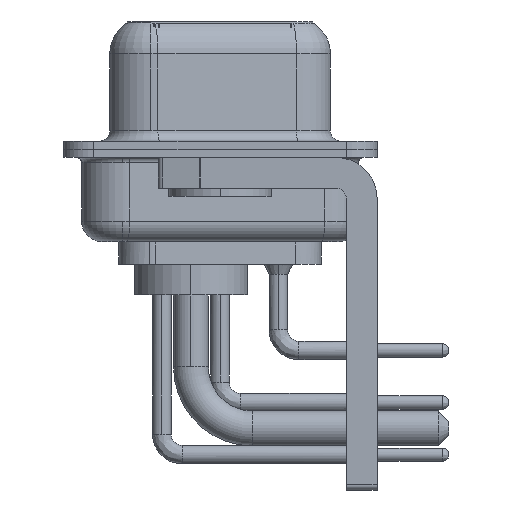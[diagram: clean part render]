
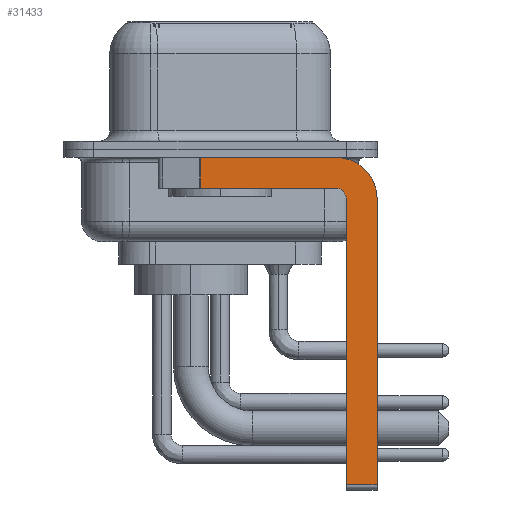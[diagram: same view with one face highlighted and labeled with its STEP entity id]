
A CAD part, left-side view. The second image highlights one B-rep face of the part: STEP entity #31433.
In plain terms, the highlighted planar face has unit normal (-1, 0, 0).
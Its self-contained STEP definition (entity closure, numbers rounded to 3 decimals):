
#426 = ORIENTED_EDGE ( 'NONE', *, *, #25855, .F. ) ;
#1283 = DIRECTION ( 'NONE',  ( 1., 0., 0. ) ) ;
#1413 = CARTESIAN_POINT ( 'NONE',  ( -2.9, 0.978, -1.9 ) ) ;
#2458 = LINE ( 'NONE', #3112, #21008 ) ;
#2875 = CIRCLE ( 'NONE', #27595, 0.5 ) ;
#3047 = CARTESIAN_POINT ( 'NONE',  ( -2.9, -5.65, -0.4 ) ) ;
#3112 = CARTESIAN_POINT ( 'NONE',  ( -2.9, -5.65, -1.9 ) ) ;
#3438 = DIRECTION ( 'NONE',  ( 1., 0., 0. ) ) ;
#4174 = LINE ( 'NONE', #7235, #6791 ) ;
#4279 = VERTEX_POINT ( 'NONE', #17895 ) ;
#5660 = CARTESIAN_POINT ( 'NONE',  ( -2.9, 0.978, -1.9 ) ) ;
#6791 = VECTOR ( 'NONE', #12461, 1000. ) ;
#7014 = ORIENTED_EDGE ( 'NONE', *, *, #28611, .F. ) ;
#7235 = CARTESIAN_POINT ( 'NONE',  ( -2.9, 3., -0.4 ) ) ;
#7258 = ORIENTED_EDGE ( 'NONE', *, *, #32996, .F. ) ;
#8480 = ORIENTED_EDGE ( 'NONE', *, *, #21871, .F. ) ;
#8624 = VERTEX_POINT ( 'NONE', #5660 ) ;
#8883 = EDGE_CURVE ( 'NONE', #15391, #8624, #19767, .T. ) ;
#9077 = EDGE_LOOP ( 'NONE', ( #7014, #14696, #9313, #30876, #8480, #16745, #426, #7258 ) ) ;
#9313 = ORIENTED_EDGE ( 'NONE', *, *, #24992, .F. ) ;
#9657 = DIRECTION ( 'NONE',  ( 0., 0., 1. ) ) ;
#9708 = CARTESIAN_POINT ( 'NONE',  ( -2.9, -5.65, -1.9 ) ) ;
#11572 = PLANE ( 'NONE',  #16784 ) ;
#12461 = DIRECTION ( 'NONE',  ( 0., -1., 0. ) ) ;
#12676 = EDGE_CURVE ( 'NONE', #21744, #14677, #2875, .T. ) ;
#14677 = VERTEX_POINT ( 'NONE', #9708 ) ;
#14696 = ORIENTED_EDGE ( 'NONE', *, *, #8883, .T. ) ;
#15271 = VERTEX_POINT ( 'NONE', #3047 ) ;
#15279 = DIRECTION ( 'NONE',  ( 0., 1., 0. ) ) ;
#15391 = VERTEX_POINT ( 'NONE', #29140 ) ;
#15447 = CARTESIAN_POINT ( 'NONE',  ( -2.9, -7.65, -2.4 ) ) ;
#15786 = CARTESIAN_POINT ( 'NONE',  ( -2.9, -5.65, -2.4 ) ) ;
#16114 = CARTESIAN_POINT ( 'NONE',  ( -2.9, -6.15, -2.4 ) ) ;
#16745 = ORIENTED_EDGE ( 'NONE', *, *, #28618, .T. ) ;
#16784 = AXIS2_PLACEMENT_3D ( 'NONE', #18979, #1283, #16798 ) ;
#16798 = DIRECTION ( 'NONE',  ( 0., 0., -1. ) ) ;
#17097 = CARTESIAN_POINT ( 'NONE',  ( -2.9, -6.15, -16.6 ) ) ;
#17416 = VERTEX_POINT ( 'NONE', #23041 ) ;
#17780 = DIRECTION ( 'NONE',  ( 0., 0., 1. ) ) ;
#17895 = CARTESIAN_POINT ( 'NONE',  ( -2.9, -7.65, -16.35 ) ) ;
#18478 = AXIS2_PLACEMENT_3D ( 'NONE', #15786, #3438, #21126 ) ;
#18798 = VECTOR ( 'NONE', #9657, 1000. ) ;
#18979 = CARTESIAN_POINT ( 'NONE',  ( -2.9, -5.65, -2.4 ) ) ;
#19395 = VECTOR ( 'NONE', #19432, 1000. ) ;
#19432 = DIRECTION ( 'NONE',  ( 0., 0., -1. ) ) ;
#19515 = DIRECTION ( 'NONE',  ( 0., -1., 0. ) ) ;
#19767 = LINE ( 'NONE', #1413, #19395 ) ;
#20124 = LINE ( 'NONE', #15447, #30247 ) ;
#21008 = VECTOR ( 'NONE', #15279, 1000. ) ;
#21126 = DIRECTION ( 'NONE',  ( 0., 0., -1. ) ) ;
#21689 = CIRCLE ( 'NONE', #18478, 2. ) ;
#21744 = VERTEX_POINT ( 'NONE', #16114 ) ;
#21871 = EDGE_CURVE ( 'NONE', #30542, #21744, #30378, .T. ) ;
#23041 = CARTESIAN_POINT ( 'NONE',  ( -2.9, -7.65, -2.4 ) ) ;
#24505 = FACE_OUTER_BOUND ( 'NONE', #9077, .T. ) ;
#24992 = EDGE_CURVE ( 'NONE', #14677, #8624, #2458, .T. ) ;
#25504 = DIRECTION ( 'NONE',  ( 0., 0., -1. ) ) ;
#25602 = VECTOR ( 'NONE', #19515, 1000. ) ;
#25855 = EDGE_CURVE ( 'NONE', #17416, #4279, #20124, .T. ) ;
#26456 = CARTESIAN_POINT ( 'NONE',  ( -2.9, -6.15, -16.35 ) ) ;
#27525 = CARTESIAN_POINT ( 'NONE',  ( -2.9, -5.65, -2.4 ) ) ;
#27595 = AXIS2_PLACEMENT_3D ( 'NONE', #27525, #30235, #17780 ) ;
#28611 = EDGE_CURVE ( 'NONE', #15391, #15271, #4174, .T. ) ;
#28618 = EDGE_CURVE ( 'NONE', #30542, #4279, #32644, .T. ) ;
#29140 = CARTESIAN_POINT ( 'NONE',  ( -2.9, 0.978, -0.4 ) ) ;
#29792 = CARTESIAN_POINT ( 'NONE',  ( -2.9, -5.65, -16.35 ) ) ;
#30235 = DIRECTION ( 'NONE',  ( -1., 0., 0. ) ) ;
#30247 = VECTOR ( 'NONE', #25504, 1000. ) ;
#30378 = LINE ( 'NONE', #17097, #18798 ) ;
#30542 = VERTEX_POINT ( 'NONE', #26456 ) ;
#30876 = ORIENTED_EDGE ( 'NONE', *, *, #12676, .F. ) ;
#31433 = ADVANCED_FACE ( 'NONE', ( #24505 ), #11572, .F. ) ;
#32644 = LINE ( 'NONE', #29792, #25602 ) ;
#32996 = EDGE_CURVE ( 'NONE', #15271, #17416, #21689, .T. ) ;
